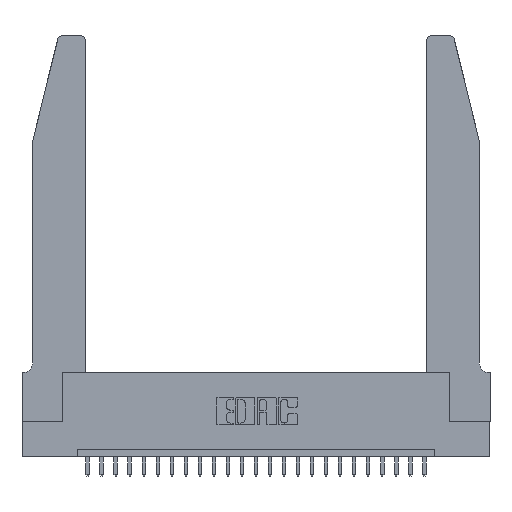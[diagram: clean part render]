
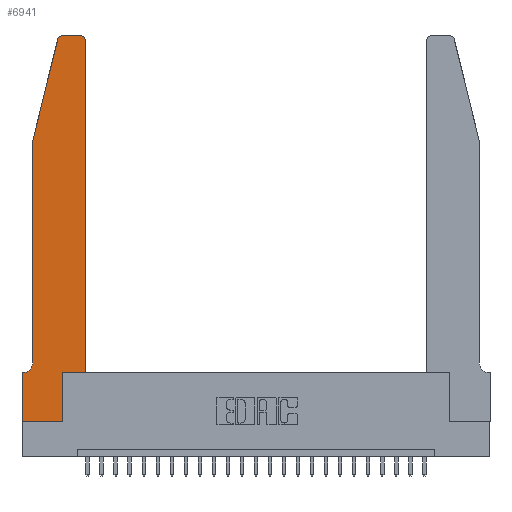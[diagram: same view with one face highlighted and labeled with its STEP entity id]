
A CAD part, top view. The second image highlights one B-rep face of the part: STEP entity #6941.
In plain terms, the highlighted planar face has unit normal (0, 0, 1).
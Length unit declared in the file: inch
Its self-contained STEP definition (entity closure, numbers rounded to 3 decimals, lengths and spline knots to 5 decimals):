
#96 = ORIENTED_EDGE ( 'NONE', *, *, #3700, .T. ) ;
#157 = LINE ( 'NONE', #17643, #13264 ) ;
#239 = CARTESIAN_POINT ( 'NONE',  ( 0.2865, 0.35, 0.37 ) ) ;
#317 = CARTESIAN_POINT ( 'NONE',  ( 0.0755, 2., 0.37 ) ) ;
#1042 = CARTESIAN_POINT ( 'NONE',  ( 0.2865, 0.35, 0.37 ) ) ;
#1374 = CARTESIAN_POINT ( 'NONE',  ( 0., 0., 0.37 ) ) ;
#1629 = VECTOR ( 'NONE', #20940, 39.37008 ) ;
#1871 = VERTEX_POINT ( 'NONE', #15697 ) ;
#1967 = CARTESIAN_POINT ( 'NONE',  ( 0., 0.35, 0.37 ) ) ;
#2017 = ORIENTED_EDGE ( 'NONE', *, *, #23950, .T. ) ;
#2021 = DIRECTION ( 'NONE',  ( -1., 0., 0. ) ) ;
#2061 = DIRECTION ( 'NONE',  ( 0., 0., 1. ) ) ;
#3083 = AXIS2_PLACEMENT_3D ( 'NONE', #1967, #2061, #24205 ) ;
#3700 = EDGE_CURVE ( 'NONE', #13432, #16067, #18605, .T. ) ;
#3716 = VECTOR ( 'NONE', #10289, 39.37008 ) ;
#4098 = DIRECTION ( 'NONE',  ( 0., 1., 0. ) ) ;
#4555 = CARTESIAN_POINT ( 'NONE',  ( 0.4205, 2.75, 0.37 ) ) ;
#4561 = CARTESIAN_POINT ( 'NONE',  ( 0., 0.35, 0.37 ) ) ;
#4804 = LINE ( 'NONE', #5397, #14421 ) ;
#5397 = CARTESIAN_POINT ( 'NONE',  ( 0.2605, 2.75, 0.37 ) ) ;
#6123 = ORIENTED_EDGE ( 'NONE', *, *, #20715, .T. ) ;
#6153 = CARTESIAN_POINT ( 'NONE',  ( 0.4205, 2.72, 0.37 ) ) ;
#6317 = VERTEX_POINT ( 'NONE', #25713 ) ;
#6941 = ADVANCED_FACE ( 'NONE', ( #16837 ), #13885, .T. ) ;
#6960 = CARTESIAN_POINT ( 'NONE',  ( 0.284, 2.75, 0.37 ) ) ;
#7098 = DIRECTION ( 'NONE',  ( 0., 1., 0. ) ) ;
#7123 = EDGE_CURVE ( 'NONE', #11998, #6317, #9045, .T. ) ;
#7339 = DIRECTION ( 'NONE',  ( -1., 0., 0. ) ) ;
#8050 = ORIENTED_EDGE ( 'NONE', *, *, #25010, .T. ) ;
#9045 = LINE ( 'NONE', #22824, #14303 ) ;
#9141 = EDGE_LOOP ( 'NONE', ( #21629, #96, #19075, #6123, #21124, #2017, #12055, #9200, #15716, #11487, #23033, #8050 ) ) ;
#9200 = ORIENTED_EDGE ( 'NONE', *, *, #23121, .T. ) ;
#9598 = CIRCLE ( 'NONE', #11835, 0.07 ) ;
#9843 = VECTOR ( 'NONE', #21294, 39.37008 ) ;
#10289 = DIRECTION ( 'NONE',  ( 0., -1., 0. ) ) ;
#10389 = EDGE_CURVE ( 'NONE', #16067, #25036, #14366, .T. ) ;
#10729 = DIRECTION ( 'NONE',  ( -1., 0., 0. ) ) ;
#11487 = ORIENTED_EDGE ( 'NONE', *, *, #7123, .T. ) ;
#11503 = VECTOR ( 'NONE', #14589, 39.37008 ) ;
#11684 = CIRCLE ( 'NONE', #17887, 0.03 ) ;
#11835 = AXIS2_PLACEMENT_3D ( 'NONE', #12879, #22677, #10729 ) ;
#11998 = VERTEX_POINT ( 'NONE', #239 ) ;
#12055 = ORIENTED_EDGE ( 'NONE', *, *, #16397, .T. ) ;
#12094 = CARTESIAN_POINT ( 'NONE',  ( 0.0755, 2., 0.37 ) ) ;
#12391 = EDGE_CURVE ( 'NONE', #6317, #23288, #20244, .T. ) ;
#12656 = CARTESIAN_POINT ( 'NONE',  ( 0.284, 2.72, 0.37 ) ) ;
#12879 = CARTESIAN_POINT ( 'NONE',  ( 0.0055, 0.42, 0.37 ) ) ;
#13264 = VECTOR ( 'NONE', #2021, 39.37008 ) ;
#13432 = VERTEX_POINT ( 'NONE', #6960 ) ;
#13885 = PLANE ( 'NONE',  #3083 ) ;
#14303 = VECTOR ( 'NONE', #14569, 39.37008 ) ;
#14366 = LINE ( 'NONE', #16256, #1629 ) ;
#14421 = VECTOR ( 'NONE', #7339, 39.37008 ) ;
#14569 = DIRECTION ( 'NONE',  ( 1., 0., 0. ) ) ;
#14589 = DIRECTION ( 'NONE',  ( 1., 0., 0. ) ) ;
#14895 = VECTOR ( 'NONE', #4098, 39.37008 ) ;
#15157 = AXIS2_PLACEMENT_3D ( 'NONE', #12656, #16558, #24882 ) ;
#15193 = VERTEX_POINT ( 'NONE', #4555 ) ;
#15478 = CARTESIAN_POINT ( 'NONE',  ( 0.2865, 0., 0.37 ) ) ;
#15489 = LINE ( 'NONE', #16713, #11503 ) ;
#15697 = CARTESIAN_POINT ( 'NONE',  ( 0.0055, 0.35, 0.37 ) ) ;
#15716 = ORIENTED_EDGE ( 'NONE', *, *, #24398, .T. ) ;
#16067 = VERTEX_POINT ( 'NONE', #24869 ) ;
#16256 = CARTESIAN_POINT ( 'NONE',  ( 0.0755, 2., 0.37 ) ) ;
#16397 = EDGE_CURVE ( 'NONE', #19643, #16998, #25780, .T. ) ;
#16558 = DIRECTION ( 'NONE',  ( 0., 0., 1. ) ) ;
#16713 = CARTESIAN_POINT ( 'NONE',  ( 0., 0., 0.37 ) ) ;
#16837 = FACE_OUTER_BOUND ( 'NONE', #9141, .T. ) ;
#16998 = VERTEX_POINT ( 'NONE', #23414 ) ;
#17109 = LINE ( 'NONE', #317, #3716 ) ;
#17643 = CARTESIAN_POINT ( 'NONE',  ( 0.0755, 0.35, 0.37 ) ) ;
#17887 = AXIS2_PLACEMENT_3D ( 'NONE', #6153, #25901, #19525 ) ;
#18605 = CIRCLE ( 'NONE', #15157, 0.03 ) ;
#19075 = ORIENTED_EDGE ( 'NONE', *, *, #10389, .T. ) ;
#19525 = DIRECTION ( 'NONE',  ( 1., 0., 0. ) ) ;
#19578 = VERTEX_POINT ( 'NONE', #19989 ) ;
#19643 = VERTEX_POINT ( 'NONE', #4561 ) ;
#19989 = CARTESIAN_POINT ( 'NONE',  ( 0.0755, 0.42, 0.37 ) ) ;
#20244 = LINE ( 'NONE', #21037, #14895 ) ;
#20464 = LINE ( 'NONE', #1042, #22004 ) ;
#20715 = EDGE_CURVE ( 'NONE', #25036, #19578, #17109, .T. ) ;
#20940 = DIRECTION ( 'NONE',  ( -0.239, -0.971, 0. ) ) ;
#20941 = EDGE_CURVE ( 'NONE', #19578, #1871, #9598, .T. ) ;
#21037 = CARTESIAN_POINT ( 'NONE',  ( 0.4505, 0.35, 0.37 ) ) ;
#21124 = ORIENTED_EDGE ( 'NONE', *, *, #20941, .T. ) ;
#21201 = CARTESIAN_POINT ( 'NONE',  ( 0.4505, 2.72, 0.37 ) ) ;
#21294 = DIRECTION ( 'NONE',  ( 0., -1., 0. ) ) ;
#21629 = ORIENTED_EDGE ( 'NONE', *, *, #24937, .T. ) ;
#22004 = VECTOR ( 'NONE', #7098, 39.37008 ) ;
#22677 = DIRECTION ( 'NONE',  ( 0., 0., -1. ) ) ;
#22824 = CARTESIAN_POINT ( 'NONE',  ( 0.4505, 0.35, 0.37 ) ) ;
#23033 = ORIENTED_EDGE ( 'NONE', *, *, #12391, .T. ) ;
#23121 = EDGE_CURVE ( 'NONE', #16998, #25020, #15489, .T. ) ;
#23288 = VERTEX_POINT ( 'NONE', #21201 ) ;
#23414 = CARTESIAN_POINT ( 'NONE',  ( 0., 0., 0.37 ) ) ;
#23950 = EDGE_CURVE ( 'NONE', #1871, #19643, #157, .T. ) ;
#24205 = DIRECTION ( 'NONE',  ( 1., 0., 0. ) ) ;
#24398 = EDGE_CURVE ( 'NONE', #25020, #11998, #20464, .T. ) ;
#24869 = CARTESIAN_POINT ( 'NONE',  ( 0.25487, 2.72718, 0.37 ) ) ;
#24882 = DIRECTION ( 'NONE',  ( 1., 0., 0. ) ) ;
#24937 = EDGE_CURVE ( 'NONE', #15193, #13432, #4804, .T. ) ;
#25010 = EDGE_CURVE ( 'NONE', #23288, #15193, #11684, .T. ) ;
#25020 = VERTEX_POINT ( 'NONE', #15478 ) ;
#25036 = VERTEX_POINT ( 'NONE', #12094 ) ;
#25713 = CARTESIAN_POINT ( 'NONE',  ( 0.4505, 0.35, 0.37 ) ) ;
#25780 = LINE ( 'NONE', #1374, #9843 ) ;
#25901 = DIRECTION ( 'NONE',  ( 0., 0., 1. ) ) ;
